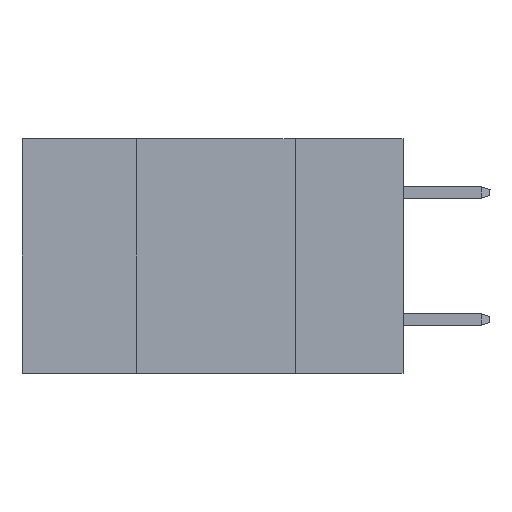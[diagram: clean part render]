
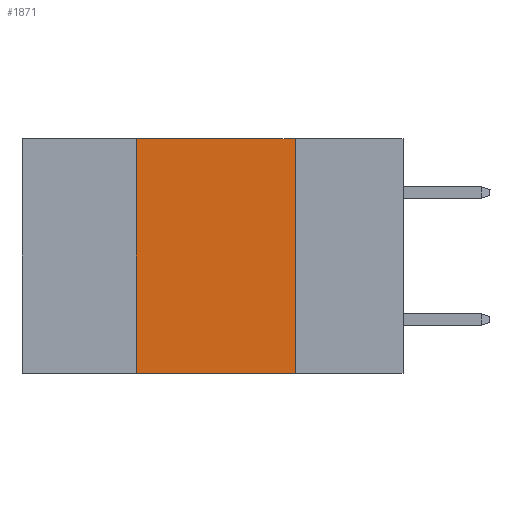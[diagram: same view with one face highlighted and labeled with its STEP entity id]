
A CAD part, left-side view. The second image highlights one B-rep face of the part: STEP entity #1871.
In plain terms, the highlighted planar face has unit normal (-1, 0, 0).
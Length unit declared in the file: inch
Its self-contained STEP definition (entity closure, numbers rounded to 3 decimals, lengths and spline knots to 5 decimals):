
#1329 = VECTOR ( 'NONE', #11737, 39.37008 ) ;
#1871 = ADVANCED_FACE ( 'NONE', ( #15399 ), #2935, .F. ) ;
#1917 = VECTOR ( 'NONE', #6786, 39.37008 ) ;
#2370 = LINE ( 'NONE', #7979, #1917 ) ;
#2522 = VERTEX_POINT ( 'NONE', #7400 ) ;
#2863 = CARTESIAN_POINT ( 'NONE',  ( 0., 0.17, 0. ) ) ;
#2935 = PLANE ( 'NONE',  #9619 ) ;
#3554 = LINE ( 'NONE', #10550, #16197 ) ;
#3575 = CARTESIAN_POINT ( 'NONE',  ( 0., 0.42, 0. ) ) ;
#3985 = ORIENTED_EDGE ( 'NONE', *, *, #4948, .F. ) ;
#4628 = EDGE_CURVE ( 'NONE', #15568, #2522, #3554, .T. ) ;
#4948 = EDGE_CURVE ( 'NONE', #10993, #2522, #11399, .T. ) ;
#5486 = ORIENTED_EDGE ( 'NONE', *, *, #8563, .F. ) ;
#5490 = VERTEX_POINT ( 'NONE', #3575 ) ;
#6786 = DIRECTION ( 'NONE',  ( 0., 0., 1. ) ) ;
#7400 = CARTESIAN_POINT ( 'NONE',  ( 0., 0.17, -0.37 ) ) ;
#7629 = VECTOR ( 'NONE', #15636, 39.37008 ) ;
#7660 = CARTESIAN_POINT ( 'NONE',  ( 0., 0.6, 0. ) ) ;
#7683 = EDGE_LOOP ( 'NONE', ( #3985, #10506, #5486, #9194 ) ) ;
#7689 = DIRECTION ( 'NONE',  ( 0., -1., 0. ) ) ;
#7979 = CARTESIAN_POINT ( 'NONE',  ( 0., 0.42, 0. ) ) ;
#8563 = EDGE_CURVE ( 'NONE', #15568, #5490, #2370, .T. ) ;
#9194 = ORIENTED_EDGE ( 'NONE', *, *, #4628, .T. ) ;
#9619 = AXIS2_PLACEMENT_3D ( 'NONE', #12435, #18060, #13826 ) ;
#10506 = ORIENTED_EDGE ( 'NONE', *, *, #16528, .F. ) ;
#10550 = CARTESIAN_POINT ( 'NONE',  ( 0., 0.6, -0.37 ) ) ;
#10993 = VERTEX_POINT ( 'NONE', #2863 ) ;
#11399 = LINE ( 'NONE', #13975, #7629 ) ;
#11737 = DIRECTION ( 'NONE',  ( 0., -1., 0. ) ) ;
#12435 = CARTESIAN_POINT ( 'NONE',  ( 0., 0.6, 0. ) ) ;
#13130 = LINE ( 'NONE', #7660, #1329 ) ;
#13826 = DIRECTION ( 'NONE',  ( 0., 0., -1. ) ) ;
#13975 = CARTESIAN_POINT ( 'NONE',  ( 0., 0.17, 0. ) ) ;
#15399 = FACE_OUTER_BOUND ( 'NONE', #7683, .T. ) ;
#15568 = VERTEX_POINT ( 'NONE', #18174 ) ;
#15636 = DIRECTION ( 'NONE',  ( 0., 0., -1. ) ) ;
#16197 = VECTOR ( 'NONE', #7689, 39.37008 ) ;
#16528 = EDGE_CURVE ( 'NONE', #5490, #10993, #13130, .T. ) ;
#18060 = DIRECTION ( 'NONE',  ( 1., 0., 0. ) ) ;
#18174 = CARTESIAN_POINT ( 'NONE',  ( 0., 0.42, -0.37 ) ) ;
